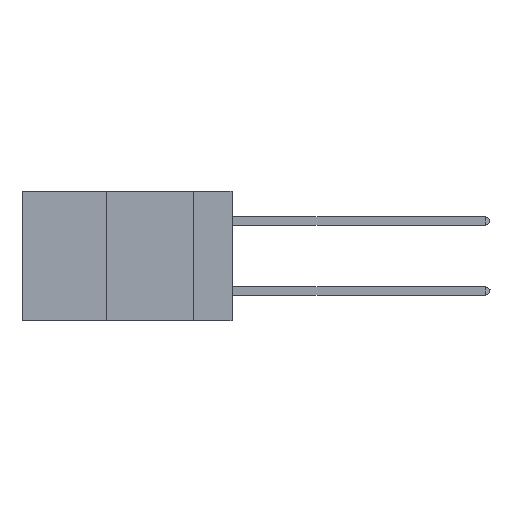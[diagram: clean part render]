
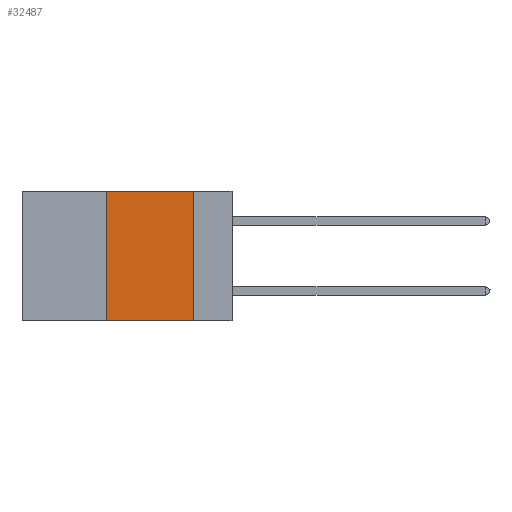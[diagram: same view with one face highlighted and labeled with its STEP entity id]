
A CAD part, left-side view. The second image highlights one B-rep face of the part: STEP entity #32487.
In plain terms, the highlighted planar face has unit normal (-1, 0, 0).
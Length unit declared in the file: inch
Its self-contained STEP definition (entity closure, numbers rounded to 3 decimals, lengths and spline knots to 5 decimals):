
#58 = CARTESIAN_POINT ( 'NONE',  ( 0., 0.11, 0. ) ) ;
#132 = LINE ( 'NONE', #27102, #1410 ) ;
#774 = EDGE_CURVE ( 'NONE', #14871, #2839, #132, .T. ) ;
#818 = DIRECTION ( 'NONE',  ( 0., 0., 1. ) ) ;
#828 = CARTESIAN_POINT ( 'NONE',  ( 0., 0.36, 0. ) ) ;
#1410 = VECTOR ( 'NONE', #2935, 39.37008 ) ;
#1461 = EDGE_CURVE ( 'NONE', #30303, #9892, #7569, .T. ) ;
#2839 = VERTEX_POINT ( 'NONE', #58 ) ;
#2935 = DIRECTION ( 'NONE',  ( 0., -1., 0. ) ) ;
#2949 = VECTOR ( 'NONE', #818, 39.37008 ) ;
#3969 = LINE ( 'NONE', #9449, #2949 ) ;
#5624 = DIRECTION ( 'NONE',  ( 0., -1., 0. ) ) ;
#6802 = DIRECTION ( 'NONE',  ( 0., 0., -1. ) ) ;
#6804 = EDGE_CURVE ( 'NONE', #30303, #14871, #3969, .T. ) ;
#6953 = CARTESIAN_POINT ( 'NONE',  ( 0., 0.6, 0. ) ) ;
#7135 = DIRECTION ( 'NONE',  ( 0., 0., -1. ) ) ;
#7569 = LINE ( 'NONE', #11090, #31917 ) ;
#9449 = CARTESIAN_POINT ( 'NONE',  ( 0., 0.36, 0. ) ) ;
#9892 = VERTEX_POINT ( 'NONE', #34734 ) ;
#10165 = EDGE_CURVE ( 'NONE', #2839, #9892, #28686, .T. ) ;
#11090 = CARTESIAN_POINT ( 'NONE',  ( 0., 0.6, -0.37 ) ) ;
#11645 = ORIENTED_EDGE ( 'NONE', *, *, #1461, .T. ) ;
#12269 = EDGE_LOOP ( 'NONE', ( #23290, #16236, #16416, #11645 ) ) ;
#14871 = VERTEX_POINT ( 'NONE', #828 ) ;
#16236 = ORIENTED_EDGE ( 'NONE', *, *, #774, .F. ) ;
#16416 = ORIENTED_EDGE ( 'NONE', *, *, #6804, .F. ) ;
#17669 = FACE_OUTER_BOUND ( 'NONE', #12269, .T. ) ;
#23290 = ORIENTED_EDGE ( 'NONE', *, *, #10165, .F. ) ;
#23613 = VECTOR ( 'NONE', #6802, 39.37008 ) ;
#25493 = CARTESIAN_POINT ( 'NONE',  ( 0., 0.11, 0. ) ) ;
#27102 = CARTESIAN_POINT ( 'NONE',  ( 0., 0.6, 0. ) ) ;
#28686 = LINE ( 'NONE', #25493, #23613 ) ;
#28743 = AXIS2_PLACEMENT_3D ( 'NONE', #6953, #30784, #7135 ) ;
#30303 = VERTEX_POINT ( 'NONE', #34029 ) ;
#30784 = DIRECTION ( 'NONE',  ( 1., 0., 0. ) ) ;
#31118 = PLANE ( 'NONE',  #28743 ) ;
#31917 = VECTOR ( 'NONE', #5624, 39.37008 ) ;
#32487 = ADVANCED_FACE ( 'NONE', ( #17669 ), #31118, .F. ) ;
#34029 = CARTESIAN_POINT ( 'NONE',  ( 0., 0.36, -0.37 ) ) ;
#34734 = CARTESIAN_POINT ( 'NONE',  ( 0., 0.11, -0.37 ) ) ;
